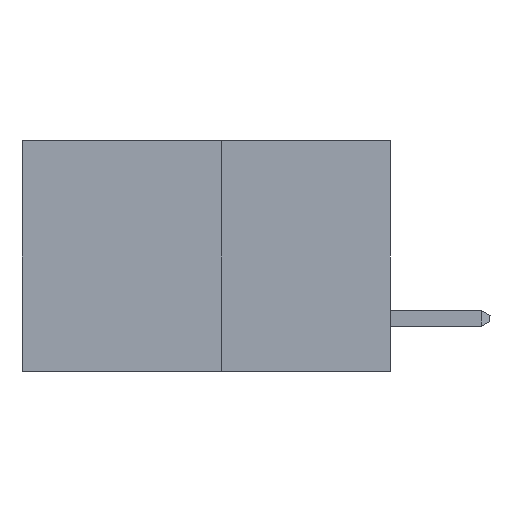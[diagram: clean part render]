
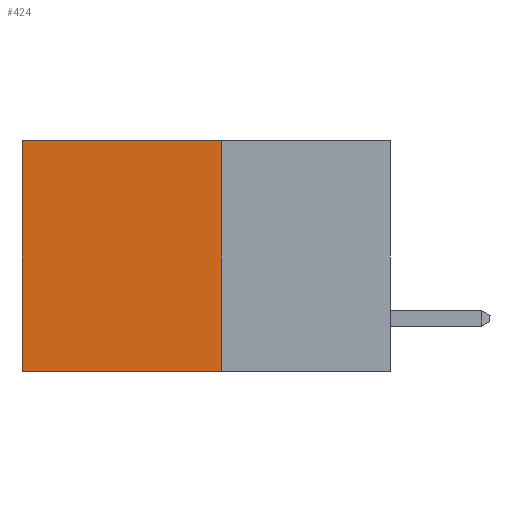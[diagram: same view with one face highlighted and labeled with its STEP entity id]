
A CAD part, left-side view. The second image highlights one B-rep face of the part: STEP entity #424.
In plain terms, the highlighted planar face has unit normal (-1, 0, 0).
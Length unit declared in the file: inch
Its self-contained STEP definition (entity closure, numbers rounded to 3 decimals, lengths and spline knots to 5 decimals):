
#121 = VECTOR ( 'NONE', #8845, 39.37008 ) ;
#240 = CARTESIAN_POINT ( 'NONE',  ( 0.277, 0.27, -0.37 ) ) ;
#418 = VERTEX_POINT ( 'NONE', #240 ) ;
#424 = ADVANCED_FACE ( 'NONE', ( #5456 ), #6482, .F. ) ;
#860 = EDGE_CURVE ( 'NONE', #10661, #4633, #2204, .T. ) ;
#879 = LINE ( 'NONE', #9216, #121 ) ;
#1181 = CARTESIAN_POINT ( 'NONE',  ( 0.277, 0.59, -0.37 ) ) ;
#1654 = VECTOR ( 'NONE', #4224, 39.37008 ) ;
#1697 = DIRECTION ( 'NONE',  ( 0., 0., -1. ) ) ;
#2204 = LINE ( 'NONE', #4478, #5024 ) ;
#2817 = EDGE_CURVE ( 'NONE', #5202, #10661, #11509, .T. ) ;
#3017 = CARTESIAN_POINT ( 'NONE',  ( 0.277, 0.59, 0. ) ) ;
#4224 = DIRECTION ( 'NONE',  ( 0., 0., -1. ) ) ;
#4370 = EDGE_CURVE ( 'NONE', #418, #4633, #879, .T. ) ;
#4478 = CARTESIAN_POINT ( 'NONE',  ( 0.277, 0.59, -0.37 ) ) ;
#4633 = VERTEX_POINT ( 'NONE', #1181 ) ;
#4932 = CARTESIAN_POINT ( 'NONE',  ( 0.277, 0.27, -0.37 ) ) ;
#5024 = VECTOR ( 'NONE', #1697, 39.37008 ) ;
#5202 = VERTEX_POINT ( 'NONE', #8072 ) ;
#5456 = FACE_OUTER_BOUND ( 'NONE', #12508, .T. ) ;
#5967 = AXIS2_PLACEMENT_3D ( 'NONE', #12754, #8487, #8434 ) ;
#6422 = ORIENTED_EDGE ( 'NONE', *, *, #6519, .F. ) ;
#6482 = PLANE ( 'NONE',  #5967 ) ;
#6519 = EDGE_CURVE ( 'NONE', #5202, #418, #10344, .T. ) ;
#6573 = ORIENTED_EDGE ( 'NONE', *, *, #2817, .T. ) ;
#8072 = CARTESIAN_POINT ( 'NONE',  ( 0.277, 0.27, 0. ) ) ;
#8434 = DIRECTION ( 'NONE',  ( 0., 0., -1. ) ) ;
#8487 = DIRECTION ( 'NONE',  ( 1., 0., 0. ) ) ;
#8682 = DIRECTION ( 'NONE',  ( 0., 1., 0. ) ) ;
#8782 = VECTOR ( 'NONE', #8682, 39.37008 ) ;
#8845 = DIRECTION ( 'NONE',  ( 0., 1., 0. ) ) ;
#9008 = CARTESIAN_POINT ( 'NONE',  ( 0.277, 0.27, 0. ) ) ;
#9216 = CARTESIAN_POINT ( 'NONE',  ( 0.277, 0.27, -0.37 ) ) ;
#10344 = LINE ( 'NONE', #4932, #1654 ) ;
#10661 = VERTEX_POINT ( 'NONE', #3017 ) ;
#11509 = LINE ( 'NONE', #9008, #8782 ) ;
#12508 = EDGE_LOOP ( 'NONE', ( #12596, #13068, #6422, #6573 ) ) ;
#12596 = ORIENTED_EDGE ( 'NONE', *, *, #860, .T. ) ;
#12754 = CARTESIAN_POINT ( 'NONE',  ( 0.277, 0.27, -0.37 ) ) ;
#13068 = ORIENTED_EDGE ( 'NONE', *, *, #4370, .F. ) ;
